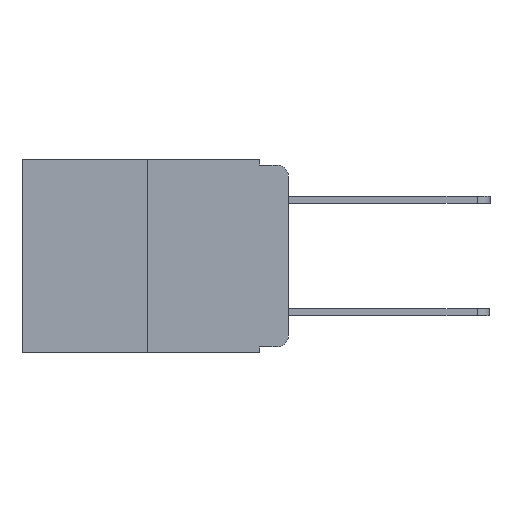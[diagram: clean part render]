
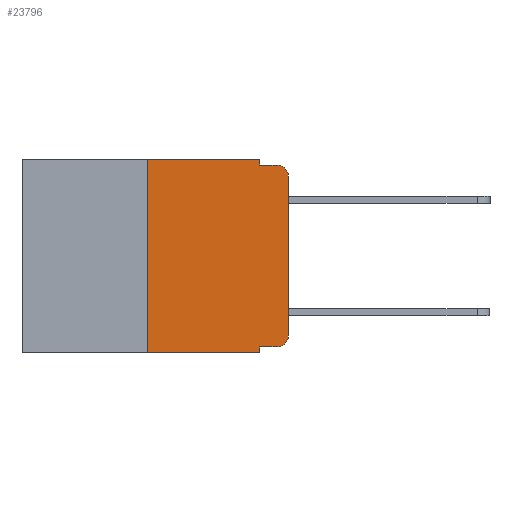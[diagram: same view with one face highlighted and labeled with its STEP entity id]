
A CAD part, left-side view. The second image highlights one B-rep face of the part: STEP entity #23796.
In plain terms, the highlighted planar face has unit normal (-1, 0, 0).
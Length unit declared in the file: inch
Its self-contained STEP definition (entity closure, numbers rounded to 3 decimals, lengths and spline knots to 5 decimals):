
#413 = VERTEX_POINT ( 'NONE', #1489 ) ;
#419 = DIRECTION ( 'NONE',  ( -1., 0., 0. ) ) ;
#445 = VERTEX_POINT ( 'NONE', #11337 ) ;
#1489 = CARTESIAN_POINT ( 'NONE',  ( 0., 0., -0.313 ) ) ;
#1885 = CARTESIAN_POINT ( 'NONE',  ( 0., 0.473, 0. ) ) ;
#2132 = ORIENTED_EDGE ( 'NONE', *, *, #21490, .T. ) ;
#2575 = VERTEX_POINT ( 'NONE', #5869 ) ;
#3264 = DIRECTION ( 'NONE',  ( 0., -1., 0. ) ) ;
#3442 = VECTOR ( 'NONE', #11790, 39.37008 ) ;
#3847 = CARTESIAN_POINT ( 'NONE',  ( 0., 0., 0. ) ) ;
#4004 = DIRECTION ( 'NONE',  ( 0., 0., 1. ) ) ;
#4141 = EDGE_CURVE ( 'NONE', #445, #2575, #8801, .T. ) ;
#4760 = ORIENTED_EDGE ( 'NONE', *, *, #13609, .T. ) ;
#5153 = CARTESIAN_POINT ( 'NONE',  ( 0., 0.051, 0. ) ) ;
#5492 = CARTESIAN_POINT ( 'NONE',  ( 0., 0.051, 0. ) ) ;
#5569 = EDGE_CURVE ( 'NONE', #2575, #413, #6839, .T. ) ;
#5856 = ORIENTED_EDGE ( 'NONE', *, *, #5569, .T. ) ;
#5869 = CARTESIAN_POINT ( 'NONE',  ( 0., 0.02, -0.333 ) ) ;
#5947 = ORIENTED_EDGE ( 'NONE', *, *, #22934, .F. ) ;
#6529 = DIRECTION ( 'NONE',  ( 0., 0., -1. ) ) ;
#6577 = EDGE_CURVE ( 'NONE', #413, #12165, #20541, .T. ) ;
#6694 = ORIENTED_EDGE ( 'NONE', *, *, #6577, .T. ) ;
#6839 = CIRCLE ( 'NONE', #17492, 0.02 ) ;
#7122 = AXIS2_PLACEMENT_3D ( 'NONE', #9517, #22555, #11535 ) ;
#7498 = ORIENTED_EDGE ( 'NONE', *, *, #13931, .F. ) ;
#8175 = VECTOR ( 'NONE', #10164, 39.37008 ) ;
#8801 = LINE ( 'NONE', #19557, #8175 ) ;
#9517 = CARTESIAN_POINT ( 'NONE',  ( 0., 0.02, -0.03 ) ) ;
#9789 = CIRCLE ( 'NONE', #7122, 0.02 ) ;
#9808 = DIRECTION ( 'NONE',  ( 0., 0., 1. ) ) ;
#9900 = VECTOR ( 'NONE', #3264, 39.37008 ) ;
#10142 = AXIS2_PLACEMENT_3D ( 'NONE', #21395, #23181, #12213 ) ;
#10164 = DIRECTION ( 'NONE',  ( 0., -1., 0. ) ) ;
#10437 = DIRECTION ( 'NONE',  ( 0., -1., 0. ) ) ;
#10656 = VECTOR ( 'NONE', #4004, 39.37008 ) ;
#10820 = CARTESIAN_POINT ( 'NONE',  ( 0., 0.25, -0.343 ) ) ;
#10908 = VERTEX_POINT ( 'NONE', #13412 ) ;
#11337 = CARTESIAN_POINT ( 'NONE',  ( 0., 0.051, -0.333 ) ) ;
#11416 = EDGE_CURVE ( 'NONE', #18628, #18267, #24607, .T. ) ;
#11535 = DIRECTION ( 'NONE',  ( 0., 0., -1. ) ) ;
#11790 = DIRECTION ( 'NONE',  ( 0., -1., 0. ) ) ;
#12165 = VERTEX_POINT ( 'NONE', #21844 ) ;
#12213 = DIRECTION ( 'NONE',  ( 0., 0., -1. ) ) ;
#12244 = VECTOR ( 'NONE', #6529, 39.37008 ) ;
#12344 = CARTESIAN_POINT ( 'NONE',  ( 0., 0.02, -0.313 ) ) ;
#12690 = LINE ( 'NONE', #5492, #17073 ) ;
#13195 = CARTESIAN_POINT ( 'NONE',  ( 0., 0.02, -0.01 ) ) ;
#13412 = CARTESIAN_POINT ( 'NONE',  ( 0., 0.051, -0.343 ) ) ;
#13609 = EDGE_CURVE ( 'NONE', #12165, #18267, #9789, .T. ) ;
#13644 = EDGE_LOOP ( 'NONE', ( #6694, #4760, #14110, #7498, #18699, #15603, #2132, #5947, #19912, #5856 ) ) ;
#13931 = EDGE_CURVE ( 'NONE', #16918, #18628, #22022, .T. ) ;
#14110 = ORIENTED_EDGE ( 'NONE', *, *, #11416, .F. ) ;
#14213 = DIRECTION ( 'NONE',  ( 0., 0., -1. ) ) ;
#14372 = CARTESIAN_POINT ( 'NONE',  ( 0., 0.051, 0. ) ) ;
#14928 = CARTESIAN_POINT ( 'NONE',  ( 0., 0.051, -0.01 ) ) ;
#15603 = ORIENTED_EDGE ( 'NONE', *, *, #23696, .F. ) ;
#15643 = CARTESIAN_POINT ( 'NONE',  ( 0., 0.25, 0. ) ) ;
#15886 = PLANE ( 'NONE',  #10142 ) ;
#16918 = VERTEX_POINT ( 'NONE', #5153 ) ;
#17073 = VECTOR ( 'NONE', #20750, 39.37008 ) ;
#17181 = FACE_OUTER_BOUND ( 'NONE', #13644, .T. ) ;
#17492 = AXIS2_PLACEMENT_3D ( 'NONE', #12344, #419, #14213 ) ;
#17980 = CARTESIAN_POINT ( 'NONE',  ( 0., 0.051, -0.01 ) ) ;
#18267 = VERTEX_POINT ( 'NONE', #13195 ) ;
#18628 = VERTEX_POINT ( 'NONE', #17980 ) ;
#18699 = ORIENTED_EDGE ( 'NONE', *, *, #19962, .F. ) ;
#19557 = CARTESIAN_POINT ( 'NONE',  ( 0., 0.051, -0.333 ) ) ;
#19811 = CARTESIAN_POINT ( 'NONE',  ( 0., 0.473, -0.343 ) ) ;
#19912 = ORIENTED_EDGE ( 'NONE', *, *, #4141, .T. ) ;
#19962 = EDGE_CURVE ( 'NONE', #22569, #16918, #23536, .T. ) ;
#19968 = VECTOR ( 'NONE', #9808, 39.37008 ) ;
#20045 = LINE ( 'NONE', #15643, #10656 ) ;
#20541 = LINE ( 'NONE', #3847, #19968 ) ;
#20750 = DIRECTION ( 'NONE',  ( 0., 0., -1. ) ) ;
#20869 = LINE ( 'NONE', #19811, #23345 ) ;
#21395 = CARTESIAN_POINT ( 'NONE',  ( 0., 0.473, 0. ) ) ;
#21490 = EDGE_CURVE ( 'NONE', #22730, #10908, #20869, .T. ) ;
#21844 = CARTESIAN_POINT ( 'NONE',  ( 0., 0., -0.03 ) ) ;
#22022 = LINE ( 'NONE', #14372, #12244 ) ;
#22555 = DIRECTION ( 'NONE',  ( -1., 0., 0. ) ) ;
#22569 = VERTEX_POINT ( 'NONE', #23187 ) ;
#22730 = VERTEX_POINT ( 'NONE', #10820 ) ;
#22934 = EDGE_CURVE ( 'NONE', #445, #10908, #12690, .T. ) ;
#23181 = DIRECTION ( 'NONE',  ( 1., 0., 0. ) ) ;
#23187 = CARTESIAN_POINT ( 'NONE',  ( 0., 0.25, 0. ) ) ;
#23345 = VECTOR ( 'NONE', #10437, 39.37008 ) ;
#23536 = LINE ( 'NONE', #1885, #3442 ) ;
#23696 = EDGE_CURVE ( 'NONE', #22730, #22569, #20045, .T. ) ;
#23796 = ADVANCED_FACE ( 'NONE', ( #17181 ), #15886, .F. ) ;
#24607 = LINE ( 'NONE', #14928, #9900 ) ;
